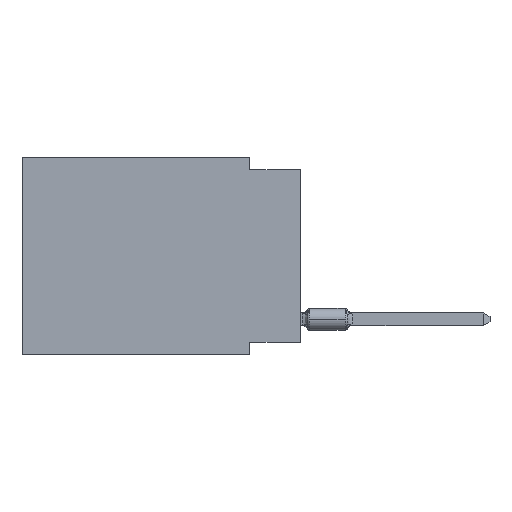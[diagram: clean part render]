
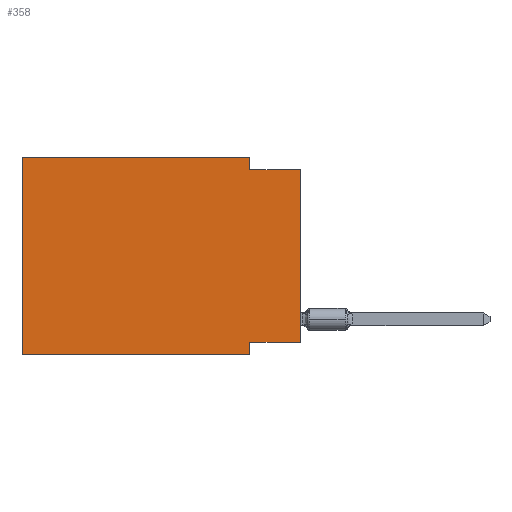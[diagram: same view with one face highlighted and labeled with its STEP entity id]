
A CAD part, left-side view. The second image highlights one B-rep face of the part: STEP entity #358.
In plain terms, the highlighted planar face has unit normal (-1, 0, 0).
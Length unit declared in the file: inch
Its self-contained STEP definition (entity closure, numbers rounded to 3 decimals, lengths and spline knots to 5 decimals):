
#358 = ADVANCED_FACE ( 'NONE', ( #6382 ), #7589, .F. ) ;
#796 = CARTESIAN_POINT ( 'NONE',  ( 0., 0., -0.365 ) ) ;
#836 = ORIENTED_EDGE ( 'NONE', *, *, #12733, .T. ) ;
#1073 = EDGE_LOOP ( 'NONE', ( #836, #2953, #4107, #1207, #7043, #13723, #2913, #9266 ) ) ;
#1163 = DIRECTION ( 'NONE',  ( 0., 0., -1. ) ) ;
#1207 = ORIENTED_EDGE ( 'NONE', *, *, #16824, .F. ) ;
#1251 = EDGE_CURVE ( 'NONE', #5546, #8657, #11536, .T. ) ;
#1314 = LINE ( 'NONE', #11741, #12829 ) ;
#2011 = VECTOR ( 'NONE', #3971, 39.37008 ) ;
#2359 = EDGE_CURVE ( 'NONE', #2653, #11561, #5093, .T. ) ;
#2653 = VERTEX_POINT ( 'NONE', #3436 ) ;
#2913 = ORIENTED_EDGE ( 'NONE', *, *, #2359, .F. ) ;
#2953 = ORIENTED_EDGE ( 'NONE', *, *, #11442, .F. ) ;
#3113 = CARTESIAN_POINT ( 'NONE',  ( 0., 0.1, -0.025 ) ) ;
#3436 = CARTESIAN_POINT ( 'NONE',  ( 0., 0.1, -0.365 ) ) ;
#3667 = CARTESIAN_POINT ( 'NONE',  ( 0., 0., -0.025 ) ) ;
#3726 = CARTESIAN_POINT ( 'NONE',  ( 0., 0., -0.365 ) ) ;
#3752 = LINE ( 'NONE', #16822, #4207 ) ;
#3971 = DIRECTION ( 'NONE',  ( 0., 1., 0. ) ) ;
#4107 = ORIENTED_EDGE ( 'NONE', *, *, #13358, .F. ) ;
#4207 = VECTOR ( 'NONE', #6229, 39.37008 ) ;
#5041 = VERTEX_POINT ( 'NONE', #796 ) ;
#5093 = LINE ( 'NONE', #10058, #14169 ) ;
#5133 = DIRECTION ( 'NONE',  ( 0., 0., 1. ) ) ;
#5401 = VECTOR ( 'NONE', #5133, 39.37008 ) ;
#5546 = VERTEX_POINT ( 'NONE', #16841 ) ;
#5942 = EDGE_CURVE ( 'NONE', #5546, #11561, #13180, .T. ) ;
#6229 = DIRECTION ( 'NONE',  ( 0., -1., 0. ) ) ;
#6308 = DIRECTION ( 'NONE',  ( 0., -1., 0. ) ) ;
#6382 = FACE_OUTER_BOUND ( 'NONE', #1073, .T. ) ;
#6685 = CARTESIAN_POINT ( 'NONE',  ( 0., 0.55, -0.39 ) ) ;
#7043 = ORIENTED_EDGE ( 'NONE', *, *, #1251, .F. ) ;
#7279 = AXIS2_PLACEMENT_3D ( 'NONE', #14073, #15611, #1163 ) ;
#7290 = CARTESIAN_POINT ( 'NONE',  ( 0., 0.1, 0. ) ) ;
#7589 = PLANE ( 'NONE',  #7279 ) ;
#8024 = LINE ( 'NONE', #9223, #15375 ) ;
#8657 = VERTEX_POINT ( 'NONE', #11407 ) ;
#8882 = LINE ( 'NONE', #3667, #15898 ) ;
#9087 = DIRECTION ( 'NONE',  ( 0., -1., 0. ) ) ;
#9098 = CARTESIAN_POINT ( 'NONE',  ( 0., 0., -0.025 ) ) ;
#9223 = CARTESIAN_POINT ( 'NONE',  ( 0., 0., 0. ) ) ;
#9266 = ORIENTED_EDGE ( 'NONE', *, *, #14356, .F. ) ;
#9481 = VERTEX_POINT ( 'NONE', #3113 ) ;
#9787 = VERTEX_POINT ( 'NONE', #7290 ) ;
#10058 = CARTESIAN_POINT ( 'NONE',  ( 0., 0.1, -0.39 ) ) ;
#11407 = CARTESIAN_POINT ( 'NONE',  ( 0., 0.55, 0. ) ) ;
#11418 = LINE ( 'NONE', #3726, #2011 ) ;
#11442 = EDGE_CURVE ( 'NONE', #9481, #16009, #8882, .T. ) ;
#11536 = LINE ( 'NONE', #16746, #5401 ) ;
#11561 = VERTEX_POINT ( 'NONE', #16820 ) ;
#11741 = CARTESIAN_POINT ( 'NONE',  ( 0., 0.1, 0. ) ) ;
#12733 = EDGE_CURVE ( 'NONE', #5041, #16009, #8024, .T. ) ;
#12778 = DIRECTION ( 'NONE',  ( 0., 0., -1. ) ) ;
#12829 = VECTOR ( 'NONE', #14390, 39.37008 ) ;
#13180 = LINE ( 'NONE', #6685, #15015 ) ;
#13358 = EDGE_CURVE ( 'NONE', #9787, #9481, #1314, .T. ) ;
#13723 = ORIENTED_EDGE ( 'NONE', *, *, #5942, .T. ) ;
#14073 = CARTESIAN_POINT ( 'NONE',  ( 0., 0.55, 0. ) ) ;
#14169 = VECTOR ( 'NONE', #12778, 39.37008 ) ;
#14344 = DIRECTION ( 'NONE',  ( 0., 0., 1. ) ) ;
#14356 = EDGE_CURVE ( 'NONE', #5041, #2653, #11418, .T. ) ;
#14390 = DIRECTION ( 'NONE',  ( 0., 0., -1. ) ) ;
#15015 = VECTOR ( 'NONE', #9087, 39.37008 ) ;
#15375 = VECTOR ( 'NONE', #14344, 39.37008 ) ;
#15611 = DIRECTION ( 'NONE',  ( 1., 0., 0. ) ) ;
#15898 = VECTOR ( 'NONE', #6308, 39.37008 ) ;
#16009 = VERTEX_POINT ( 'NONE', #9098 ) ;
#16746 = CARTESIAN_POINT ( 'NONE',  ( 0., 0.55, 0. ) ) ;
#16820 = CARTESIAN_POINT ( 'NONE',  ( 0., 0.1, -0.39 ) ) ;
#16822 = CARTESIAN_POINT ( 'NONE',  ( 0., 0.55, 0. ) ) ;
#16824 = EDGE_CURVE ( 'NONE', #8657, #9787, #3752, .T. ) ;
#16841 = CARTESIAN_POINT ( 'NONE',  ( 0., 0.55, -0.39 ) ) ;
